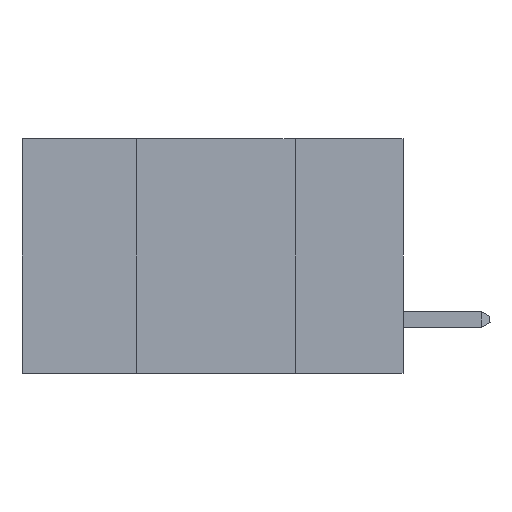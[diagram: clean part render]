
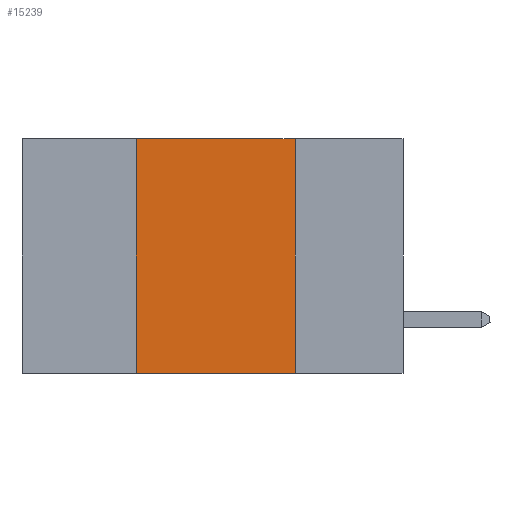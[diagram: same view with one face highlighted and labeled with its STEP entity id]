
A CAD part, left-side view. The second image highlights one B-rep face of the part: STEP entity #15239.
In plain terms, the highlighted planar face has unit normal (-1, 0, 0).
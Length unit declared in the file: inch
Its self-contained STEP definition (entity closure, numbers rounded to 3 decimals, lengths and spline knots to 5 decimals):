
#74 = CARTESIAN_POINT ( 'NONE',  ( 0., 0.17, 0. ) ) ;
#617 = CARTESIAN_POINT ( 'NONE',  ( 0., 0.6, 0. ) ) ;
#859 = CARTESIAN_POINT ( 'NONE',  ( 0., 0.6, 0. ) ) ;
#1753 = CARTESIAN_POINT ( 'NONE',  ( 0., 0.6, -0.37 ) ) ;
#2389 = CARTESIAN_POINT ( 'NONE',  ( 0., 0.42, 0. ) ) ;
#2461 = AXIS2_PLACEMENT_3D ( 'NONE', #859, #3982, #13982 ) ;
#3403 = VECTOR ( 'NONE', #21134, 39.37008 ) ;
#3982 = DIRECTION ( 'NONE',  ( 1., 0., 0. ) ) ;
#5136 = EDGE_CURVE ( 'NONE', #7664, #16188, #18038, .T. ) ;
#5169 = CARTESIAN_POINT ( 'NONE',  ( 0., 0.42, -0.37 ) ) ;
#5508 = ORIENTED_EDGE ( 'NONE', *, *, #5136, .F. ) ;
#5739 = ORIENTED_EDGE ( 'NONE', *, *, #9494, .F. ) ;
#6126 = EDGE_CURVE ( 'NONE', #15509, #18746, #15706, .T. ) ;
#6443 = EDGE_CURVE ( 'NONE', #16188, #18746, #15952, .T. ) ;
#6964 = CARTESIAN_POINT ( 'NONE',  ( 0., 0.17, 0. ) ) ;
#7064 = CARTESIAN_POINT ( 'NONE',  ( 0., 0.17, -0.37 ) ) ;
#7664 = VERTEX_POINT ( 'NONE', #7806 ) ;
#7806 = CARTESIAN_POINT ( 'NONE',  ( 0., 0.42, 0. ) ) ;
#9494 = EDGE_CURVE ( 'NONE', #15509, #7664, #19950, .T. ) ;
#10980 = VECTOR ( 'NONE', #18492, 39.37008 ) ;
#11614 = DIRECTION ( 'NONE',  ( 0., -1., 0. ) ) ;
#12048 = DIRECTION ( 'NONE',  ( 0., -1., 0. ) ) ;
#13383 = VECTOR ( 'NONE', #11614, 39.37008 ) ;
#13982 = DIRECTION ( 'NONE',  ( 0., 0., -1. ) ) ;
#14780 = EDGE_LOOP ( 'NONE', ( #20246, #5508, #5739, #18357 ) ) ;
#15239 = ADVANCED_FACE ( 'NONE', ( #20966 ), #16797, .F. ) ;
#15509 = VERTEX_POINT ( 'NONE', #5169 ) ;
#15706 = LINE ( 'NONE', #1753, #13383 ) ;
#15952 = LINE ( 'NONE', #74, #3403 ) ;
#16188 = VERTEX_POINT ( 'NONE', #6964 ) ;
#16797 = PLANE ( 'NONE',  #2461 ) ;
#17291 = VECTOR ( 'NONE', #12048, 39.37008 ) ;
#18038 = LINE ( 'NONE', #617, #17291 ) ;
#18357 = ORIENTED_EDGE ( 'NONE', *, *, #6126, .T. ) ;
#18492 = DIRECTION ( 'NONE',  ( 0., 0., 1. ) ) ;
#18746 = VERTEX_POINT ( 'NONE', #7064 ) ;
#19950 = LINE ( 'NONE', #2389, #10980 ) ;
#20246 = ORIENTED_EDGE ( 'NONE', *, *, #6443, .F. ) ;
#20966 = FACE_OUTER_BOUND ( 'NONE', #14780, .T. ) ;
#21134 = DIRECTION ( 'NONE',  ( 0., 0., -1. ) ) ;
